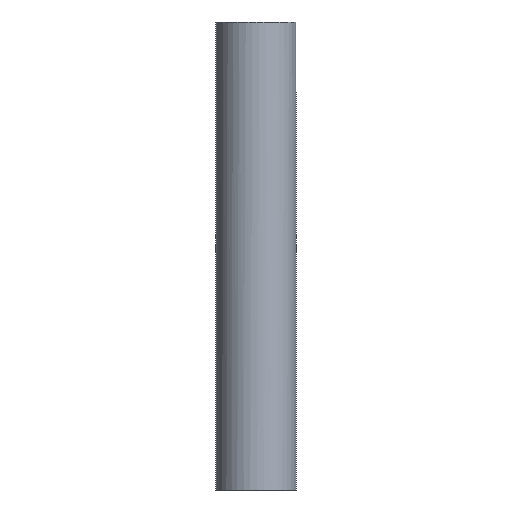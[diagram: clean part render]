
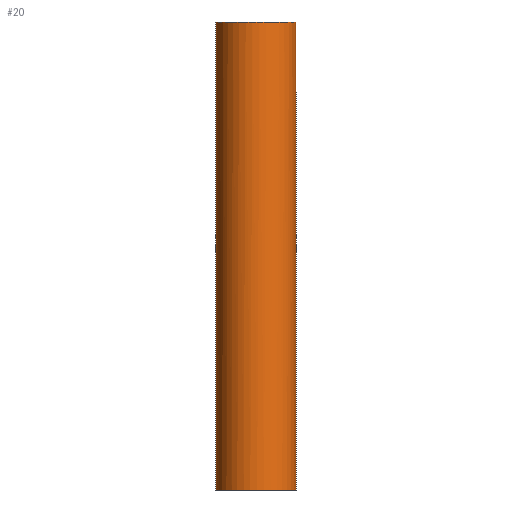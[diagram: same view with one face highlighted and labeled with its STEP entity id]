
A CAD part, front view. The second image highlights one B-rep face of the part: STEP entity #20.
In plain terms, the highlighted cylindrical face has radius 17.513 mm (diameter 35.027 mm), a full revolution.
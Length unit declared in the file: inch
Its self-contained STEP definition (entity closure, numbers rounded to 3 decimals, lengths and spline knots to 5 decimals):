
#3 = VERTEX_POINT ( 'NONE', #229 ) ;
#4 = VERTEX_POINT ( 'NONE', #51 ) ;
#12 = CYLINDRICAL_SURFACE ( 'NONE', #29, 0.6895 ) ;
#15 = CARTESIAN_POINT ( 'NONE',  ( 0., 0., 8.035 ) ) ;
#18 = DIRECTION ( 'NONE',  ( 0., 0., 1. ) ) ;
#20 = ADVANCED_FACE ( 'NONE', ( #23, #260 ), #12, .T. ) ;
#21 = CARTESIAN_POINT ( 'NONE',  ( -0.00831, 0.68946, 7.89191 ) ) ;
#22 = CARTESIAN_POINT ( 'NONE',  ( -0.0635, 0.68657, 7.955 ) ) ;
#23 = FACE_OUTER_BOUND ( 'NONE', #265, .T. ) ;
#24 = ORIENTED_EDGE ( 'NONE', *, *, #198, .F. ) ;
#29 = AXIS2_PLACEMENT_3D ( 'NONE', #239, #123, #30 ) ;
#30 = DIRECTION ( 'NONE',  ( -1., 0., 0. ) ) ;
#40 = DIRECTION ( 'NONE',  ( 1., 0., 0. ) ) ;
#42 = CARTESIAN_POINT ( 'NONE',  ( -0.0635, 0.68657, 8.035 ) ) ;
#43 = CARTESIAN_POINT ( 'NONE',  ( 0.06147, 0.68675, 7.93856 ) ) ;
#46 = CARTESIAN_POINT ( 'NONE',  ( -0.02041, 0.68921, 7.89473 ) ) ;
#51 = CARTESIAN_POINT ( 'NONE',  ( 0.0635, 0.68657, 7.955 ) ) ;
#65 = CARTESIAN_POINT ( 'NONE',  ( 0.05706, 0.68714, 7.92684 ) ) ;
#66 = CARTESIAN_POINT ( 'NONE',  ( -0.03182, 0.68877, 7.89989 ) ) ;
#85 = CIRCLE ( 'NONE', #141, 0.6895 ) ;
#88 = CARTESIAN_POINT ( 'NONE',  ( 0.05051, 0.68765, 7.91629 ) ) ;
#89 = CARTESIAN_POINT ( 'NONE',  ( -0.0419, 0.68823, 7.90711 ) ) ;
#107 = CARTESIAN_POINT ( 'NONE',  ( -0.0635, 0.68657, 8.035 ) ) ;
#110 = CARTESIAN_POINT ( 'NONE',  ( 0.03905, 0.68842, 7.90424 ) ) ;
#113 = CARTESIAN_POINT ( 'NONE',  ( -0.05046, 0.68765, 7.91624 ) ) ;
#118 = EDGE_LOOP ( 'NONE', ( #294, #24, #119, #281 ) ) ;
#119 = ORIENTED_EDGE ( 'NONE', *, *, #268, .F. ) ;
#123 = DIRECTION ( 'NONE',  ( 0., 0., -1. ) ) ;
#134 = DIRECTION ( 'NONE',  ( 0., 0., 1. ) ) ;
#136 = CARTESIAN_POINT ( 'NONE',  ( 0.01669, 0.68934, 7.89318 ) ) ;
#137 = CARTESIAN_POINT ( 'NONE',  ( -0.05706, 0.68714, 7.92682 ) ) ;
#141 = AXIS2_PLACEMENT_3D ( 'NONE', #272, #134, #291 ) ;
#144 = VERTEX_POINT ( 'NONE', #289 ) ;
#147 = LINE ( 'NONE', #209, #258 ) ;
#157 = CARTESIAN_POINT ( 'NONE',  ( 0.0635, 0.68657, 8.035 ) ) ;
#162 = DIRECTION ( 'NONE',  ( 0., 0., -1. ) ) ;
#163 = CARTESIAN_POINT ( 'NONE',  ( 0.0635, 0.68657, 7.955 ) ) ;
#164 = CARTESIAN_POINT ( 'NONE',  ( -0.0041, 0.6895, 7.8915 ) ) ;
#167 = CARTESIAN_POINT ( 'NONE',  ( -0.0635, 0.68657, 7.94661 ) ) ;
#174 = AXIS2_PLACEMENT_3D ( 'NONE', #15, #184, #40 ) ;
#178 = ORIENTED_EDGE ( 'NONE', *, *, #227, .T. ) ;
#184 = DIRECTION ( 'NONE',  ( 0., 0., 1. ) ) ;
#185 = VERTEX_POINT ( 'NONE', #107 ) ;
#186 = CARTESIAN_POINT ( 'NONE',  ( 0.06309, 0.68661, 7.94668 ) ) ;
#187 = CARTESIAN_POINT ( 'NONE',  ( -0.01645, 0.68932, 7.89353 ) ) ;
#198 = EDGE_CURVE ( 'NONE', #185, #200, #279, .T. ) ;
#200 = VERTEX_POINT ( 'NONE', #157 ) ;
#207 = B_SPLINE_CURVE_WITH_KNOTS ( 'NONE', 3,
 ( #163, #293, #186, #43, #211, #65, #230, #88, #252, #110, #274, #136, #296, #164, #21, #187, #46, #212, #66, #232, #89, #253, #113, #276, #137, #297, #167, #22 ),
 .UNSPECIFIED., .F., .F.,
 ( 4, 2, 2, 2, 2, 2, 2, 2, 2, 2, 2, 2, 2, 4 ),
 ( 0., 0.00032, 0.00063, 0.00095, 0.00126, 0.00189, 0.00252, 0.00284, 0.00315, 0.00347, 0.00378, 0.0041, 0.00441, 0.00504 ),
 .UNSPECIFIED. ) ;
#209 = CARTESIAN_POINT ( 'NONE',  ( 0.0635, 0.68657, 8.035 ) ) ;
#211 = CARTESIAN_POINT ( 'NONE',  ( 0.06025, 0.68686, 7.93453 ) ) ;
#212 = CARTESIAN_POINT ( 'NONE',  ( -0.0281, 0.68894, 7.8979 ) ) ;
#227 = EDGE_CURVE ( 'NONE', #3, #3, #85, .T. ) ;
#229 = CARTESIAN_POINT ( 'NONE',  ( 0.6895, 0., 0. ) ) ;
#230 = CARTESIAN_POINT ( 'NONE',  ( 0.05511, 0.6873, 7.92319 ) ) ;
#232 = CARTESIAN_POINT ( 'NONE',  ( -0.0387, 0.68842, 7.90448 ) ) ;
#238 = EDGE_CURVE ( 'NONE', #200, #4, #147, .T. ) ;
#239 = CARTESIAN_POINT ( 'NONE',  ( 0., 0., 8.035 ) ) ;
#248 = VECTOR ( 'NONE', #18, 39.37008 ) ;
#252 = CARTESIAN_POINT ( 'NONE',  ( 0.04783, 0.68785, 7.91302 ) ) ;
#253 = CARTESIAN_POINT ( 'NONE',  ( -0.04784, 0.68785, 7.91303 ) ) ;
#258 = VECTOR ( 'NONE', #162, 39.37008 ) ;
#260 = FACE_OUTER_BOUND ( 'NONE', #118, .T. ) ;
#261 = LINE ( 'NONE', #42, #248 ) ;
#265 = EDGE_LOOP ( 'NONE', ( #178 ) ) ;
#268 = EDGE_CURVE ( 'NONE', #144, #185, #261, .T. ) ;
#272 = CARTESIAN_POINT ( 'NONE',  ( 0., 0., 0. ) ) ;
#274 = CARTESIAN_POINT ( 'NONE',  ( 0.03197, 0.6888, 7.89951 ) ) ;
#276 = CARTESIAN_POINT ( 'NONE',  ( -0.05507, 0.6873, 7.92311 ) ) ;
#279 = CIRCLE ( 'NONE', #174, 0.6895 ) ;
#281 = ORIENTED_EDGE ( 'NONE', *, *, #282, .F. ) ;
#282 = EDGE_CURVE ( 'NONE', #4, #144, #207, .T. ) ;
#289 = CARTESIAN_POINT ( 'NONE',  ( -0.0635, 0.68657, 7.955 ) ) ;
#291 = DIRECTION ( 'NONE',  ( 1., 0., 0. ) ) ;
#293 = CARTESIAN_POINT ( 'NONE',  ( 0.0635, 0.68657, 7.9508 ) ) ;
#294 = ORIENTED_EDGE ( 'NONE', *, *, #238, .F. ) ;
#296 = CARTESIAN_POINT ( 'NONE',  ( 0.00833, 0.6895, 7.89151 ) ) ;
#297 = CARTESIAN_POINT ( 'NONE',  ( -0.06184, 0.68673, 7.93835 ) ) ;
